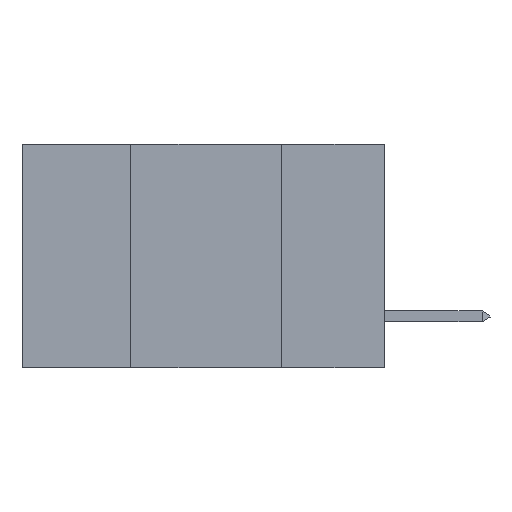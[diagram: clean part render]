
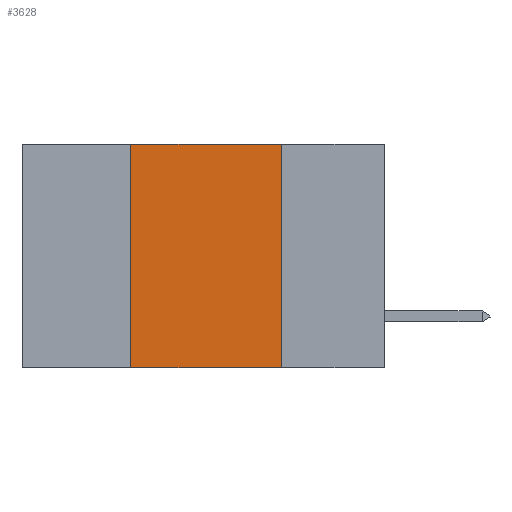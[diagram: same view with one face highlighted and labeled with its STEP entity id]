
A CAD part, left-side view. The second image highlights one B-rep face of the part: STEP entity #3628.
In plain terms, the highlighted planar face has unit normal (-1, 0, 0).
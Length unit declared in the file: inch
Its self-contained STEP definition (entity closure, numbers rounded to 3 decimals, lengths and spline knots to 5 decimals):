
#177 = DIRECTION ( 'NONE',  ( 1., 0., 0. ) ) ;
#3534 = ORIENTED_EDGE ( 'NONE', *, *, #18645, .F. ) ;
#3628 = ADVANCED_FACE ( 'NONE', ( #23068 ), #12133, .F. ) ;
#4374 = ORIENTED_EDGE ( 'NONE', *, *, #13482, .F. ) ;
#4545 = CARTESIAN_POINT ( 'NONE',  ( 0., 0.17, 0. ) ) ;
#4555 = VECTOR ( 'NONE', #10369, 39.37008 ) ;
#6362 = DIRECTION ( 'NONE',  ( 0., 0., -1. ) ) ;
#6768 = LINE ( 'NONE', #20791, #7096 ) ;
#6911 = CARTESIAN_POINT ( 'NONE',  ( 0., 0.42, -0.37 ) ) ;
#7096 = VECTOR ( 'NONE', #24781, 39.37008 ) ;
#9908 = CARTESIAN_POINT ( 'NONE',  ( 0., 0.17, 0. ) ) ;
#10297 = VECTOR ( 'NONE', #10917, 39.37008 ) ;
#10323 = ORIENTED_EDGE ( 'NONE', *, *, #13758, .F. ) ;
#10369 = DIRECTION ( 'NONE',  ( 0., 0., 1. ) ) ;
#10917 = DIRECTION ( 'NONE',  ( 0., -1., 0. ) ) ;
#12133 = PLANE ( 'NONE',  #14425 ) ;
#12821 = CARTESIAN_POINT ( 'NONE',  ( 0., 0.6, -0.37 ) ) ;
#12824 = DIRECTION ( 'NONE',  ( 0., 0., -1. ) ) ;
#13439 = VERTEX_POINT ( 'NONE', #14013 ) ;
#13482 = EDGE_CURVE ( 'NONE', #16590, #15788, #14438, .T. ) ;
#13758 = EDGE_CURVE ( 'NONE', #13856, #13439, #17268, .T. ) ;
#13856 = VERTEX_POINT ( 'NONE', #4545 ) ;
#14013 = CARTESIAN_POINT ( 'NONE',  ( 0., 0.17, -0.37 ) ) ;
#14425 = AXIS2_PLACEMENT_3D ( 'NONE', #16203, #177, #6362 ) ;
#14438 = LINE ( 'NONE', #16618, #4555 ) ;
#14490 = CARTESIAN_POINT ( 'NONE',  ( 0., 0.42, 0. ) ) ;
#14704 = ORIENTED_EDGE ( 'NONE', *, *, #21787, .T. ) ;
#15788 = VERTEX_POINT ( 'NONE', #14490 ) ;
#16203 = CARTESIAN_POINT ( 'NONE',  ( 0., 0.6, 0. ) ) ;
#16590 = VERTEX_POINT ( 'NONE', #6911 ) ;
#16618 = CARTESIAN_POINT ( 'NONE',  ( 0., 0.42, 0. ) ) ;
#17268 = LINE ( 'NONE', #9908, #20069 ) ;
#18645 = EDGE_CURVE ( 'NONE', #15788, #13856, #6768, .T. ) ;
#20069 = VECTOR ( 'NONE', #12824, 39.37008 ) ;
#20791 = CARTESIAN_POINT ( 'NONE',  ( 0., 0.6, 0. ) ) ;
#21787 = EDGE_CURVE ( 'NONE', #16590, #13439, #24927, .T. ) ;
#23043 = EDGE_LOOP ( 'NONE', ( #10323, #3534, #4374, #14704 ) ) ;
#23068 = FACE_OUTER_BOUND ( 'NONE', #23043, .T. ) ;
#24781 = DIRECTION ( 'NONE',  ( 0., -1., 0. ) ) ;
#24927 = LINE ( 'NONE', #12821, #10297 ) ;
